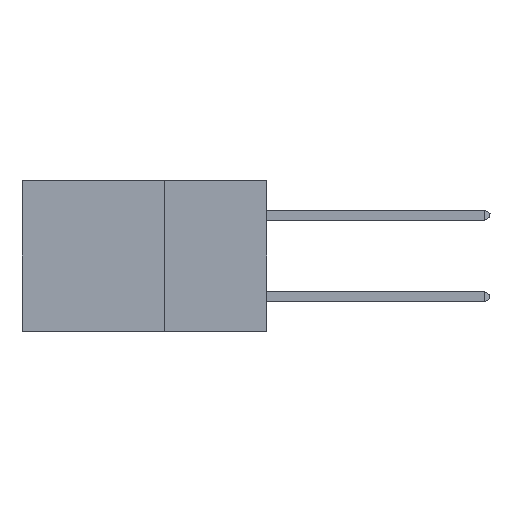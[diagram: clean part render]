
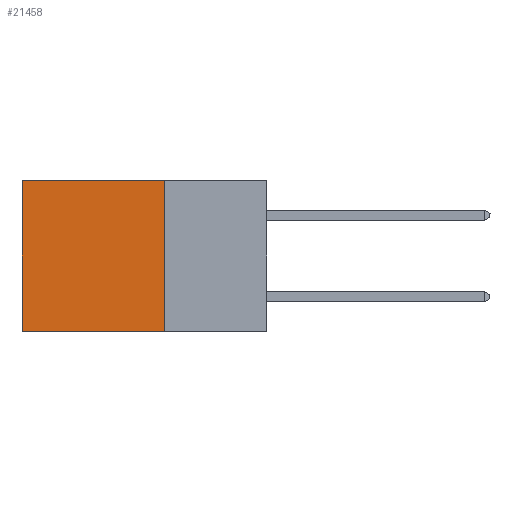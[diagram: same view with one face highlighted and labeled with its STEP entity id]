
A CAD part, left-side view. The second image highlights one B-rep face of the part: STEP entity #21458.
In plain terms, the highlighted planar face has unit normal (-1, 0, 0).
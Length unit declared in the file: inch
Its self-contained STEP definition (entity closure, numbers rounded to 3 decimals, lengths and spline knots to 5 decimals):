
#339 = EDGE_LOOP ( 'NONE', ( #19951, #11937, #10972, #16796 ) ) ;
#591 = DIRECTION ( 'NONE',  ( 0., 0., -1. ) ) ;
#736 = PLANE ( 'NONE',  #1686 ) ;
#1686 = AXIS2_PLACEMENT_3D ( 'NONE', #14239, #2355, #2596 ) ;
#2180 = CARTESIAN_POINT ( 'NONE',  ( 0.2875, 0.6, -0.37 ) ) ;
#2238 = LINE ( 'NONE', #14984, #11948 ) ;
#2355 = DIRECTION ( 'NONE',  ( 1., 0., 0. ) ) ;
#2596 = DIRECTION ( 'NONE',  ( 0., 0., -1. ) ) ;
#2606 = VERTEX_POINT ( 'NONE', #7241 ) ;
#4130 = CARTESIAN_POINT ( 'NONE',  ( 0.2875, 0.25, -0.37 ) ) ;
#4571 = VERTEX_POINT ( 'NONE', #2180 ) ;
#5546 = VERTEX_POINT ( 'NONE', #20536 ) ;
#5645 = VECTOR ( 'NONE', #8076, 39.37008 ) ;
#5891 = CARTESIAN_POINT ( 'NONE',  ( 0.2875, 0.25, 0. ) ) ;
#7241 = CARTESIAN_POINT ( 'NONE',  ( 0.2875, 0.6, 0. ) ) ;
#7673 = EDGE_CURVE ( 'NONE', #11697, #4571, #10456, .T. ) ;
#8076 = DIRECTION ( 'NONE',  ( 0., 1., 0. ) ) ;
#8188 = VECTOR ( 'NONE', #591, 39.37008 ) ;
#9347 = EDGE_CURVE ( 'NONE', #5546, #11697, #2238, .T. ) ;
#10456 = LINE ( 'NONE', #4130, #5645 ) ;
#10972 = ORIENTED_EDGE ( 'NONE', *, *, #9347, .F. ) ;
#11697 = VERTEX_POINT ( 'NONE', #14805 ) ;
#11937 = ORIENTED_EDGE ( 'NONE', *, *, #7673, .F. ) ;
#11948 = VECTOR ( 'NONE', #16575, 39.37008 ) ;
#12040 = LINE ( 'NONE', #5891, #23918 ) ;
#12814 = FACE_OUTER_BOUND ( 'NONE', #339, .T. ) ;
#12956 = EDGE_CURVE ( 'NONE', #5546, #2606, #12040, .T. ) ;
#14010 = CARTESIAN_POINT ( 'NONE',  ( 0.2875, 0.6, 0. ) ) ;
#14239 = CARTESIAN_POINT ( 'NONE',  ( 0.2875, 0.25, 0. ) ) ;
#14271 = LINE ( 'NONE', #14010, #8188 ) ;
#14805 = CARTESIAN_POINT ( 'NONE',  ( 0.2875, 0.25, -0.37 ) ) ;
#14984 = CARTESIAN_POINT ( 'NONE',  ( 0.2875, 0.25, 0. ) ) ;
#16575 = DIRECTION ( 'NONE',  ( 0., 0., -1. ) ) ;
#16796 = ORIENTED_EDGE ( 'NONE', *, *, #12956, .T. ) ;
#19382 = DIRECTION ( 'NONE',  ( 0., 1., 0. ) ) ;
#19951 = ORIENTED_EDGE ( 'NONE', *, *, #22555, .T. ) ;
#20536 = CARTESIAN_POINT ( 'NONE',  ( 0.2875, 0.25, 0. ) ) ;
#21458 = ADVANCED_FACE ( 'NONE', ( #12814 ), #736, .F. ) ;
#22555 = EDGE_CURVE ( 'NONE', #2606, #4571, #14271, .T. ) ;
#23918 = VECTOR ( 'NONE', #19382, 39.37008 ) ;
